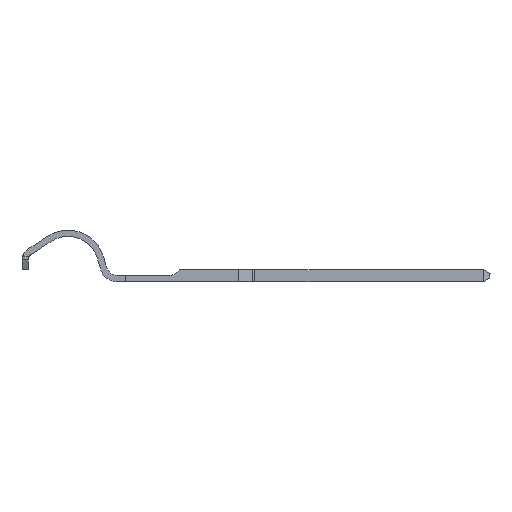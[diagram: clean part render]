
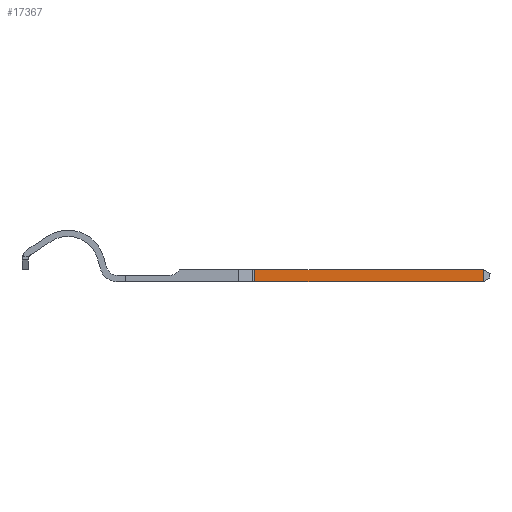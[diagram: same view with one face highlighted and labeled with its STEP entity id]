
A CAD part, left-side view. The second image highlights one B-rep face of the part: STEP entity #17367.
In plain terms, the highlighted face is planar.
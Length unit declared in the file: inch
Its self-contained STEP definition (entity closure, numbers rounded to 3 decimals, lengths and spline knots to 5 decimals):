
#159 = CARTESIAN_POINT ( 'NONE',  ( 1.08521, 0.0375, 0.0125 ) ) ;
#402 = DIRECTION ( 'NONE',  ( 1., 0., 0. ) ) ;
#1556 = CARTESIAN_POINT ( 'NONE',  ( 0.61321, -0.50791, 0.0125 ) ) ;
#2195 = VERTEX_POINT ( 'NONE', #159 ) ;
#2680 = VERTEX_POINT ( 'NONE', #18438 ) ;
#3149 = AXIS2_PLACEMENT_3D ( 'NONE', #1556, #10136, #14557 ) ;
#3330 = CARTESIAN_POINT ( 'NONE',  ( 0.61321, -0.50791, 0.0125 ) ) ;
#3728 = DIRECTION ( 'NONE',  ( 0., 1., 0. ) ) ;
#5307 = VECTOR ( 'NONE', #16184, 39.37008 ) ;
#6678 = LINE ( 'NONE', #9986, #22328 ) ;
#8253 = VERTEX_POINT ( 'NONE', #20566 ) ;
#8730 = ORIENTED_EDGE ( 'NONE', *, *, #25496, .T. ) ;
#9284 = ORIENTED_EDGE ( 'NONE', *, *, #12212, .T. ) ;
#9541 = FACE_OUTER_BOUND ( 'NONE', #26912, .T. ) ;
#9621 = EDGE_CURVE ( 'NONE', #8253, #2195, #6678, .T. ) ;
#9986 = CARTESIAN_POINT ( 'NONE',  ( 0.61321, 0.0375, 0.0125 ) ) ;
#10004 = VECTOR ( 'NONE', #3728, 39.37008 ) ;
#10136 = DIRECTION ( 'NONE',  ( 0., 0., 1. ) ) ;
#10233 = PLANE ( 'NONE',  #3149 ) ;
#10333 = ORIENTED_EDGE ( 'NONE', *, *, #9621, .F. ) ;
#11053 = VECTOR ( 'NONE', #402, 39.37008 ) ;
#12146 = DIRECTION ( 'NONE',  ( 1., 0., 0. ) ) ;
#12212 = EDGE_CURVE ( 'NONE', #2680, #2195, #15040, .T. ) ;
#14557 = DIRECTION ( 'NONE',  ( 1., 0., 0. ) ) ;
#15040 = LINE ( 'NONE', #16580, #10004 ) ;
#16184 = DIRECTION ( 'NONE',  ( 0., 1., 0. ) ) ;
#16580 = CARTESIAN_POINT ( 'NONE',  ( 1.08521, -0.50791, 0.0125 ) ) ;
#16745 = LINE ( 'NONE', #19611, #11053 ) ;
#17367 = ADVANCED_FACE ( 'NONE', ( #9541 ), #10233, .T. ) ;
#18438 = CARTESIAN_POINT ( 'NONE',  ( 1.08521, 0.0125, 0.0125 ) ) ;
#19611 = CARTESIAN_POINT ( 'NONE',  ( 0.61321, 0.0125, 0.0125 ) ) ;
#20364 = ORIENTED_EDGE ( 'NONE', *, *, #21614, .F. ) ;
#20566 = CARTESIAN_POINT ( 'NONE',  ( 0.61321, 0.0375, 0.0125 ) ) ;
#21614 = EDGE_CURVE ( 'NONE', #25124, #8253, #27157, .T. ) ;
#22328 = VECTOR ( 'NONE', #12146, 39.37008 ) ;
#22535 = CARTESIAN_POINT ( 'NONE',  ( 0.61321, 0.0125, 0.0125 ) ) ;
#25124 = VERTEX_POINT ( 'NONE', #22535 ) ;
#25496 = EDGE_CURVE ( 'NONE', #25124, #2680, #16745, .T. ) ;
#26912 = EDGE_LOOP ( 'NONE', ( #8730, #9284, #10333, #20364 ) ) ;
#27157 = LINE ( 'NONE', #3330, #5307 ) ;
